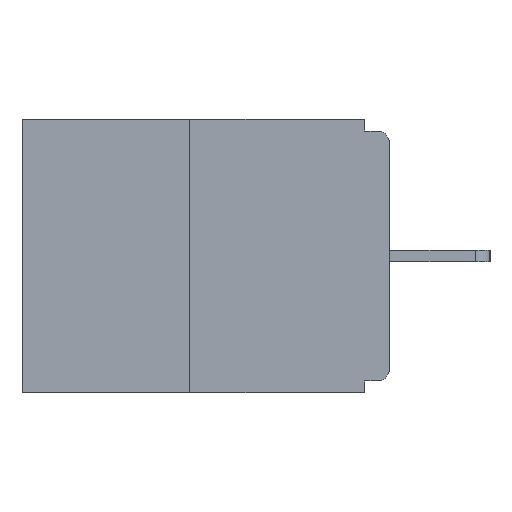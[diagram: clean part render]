
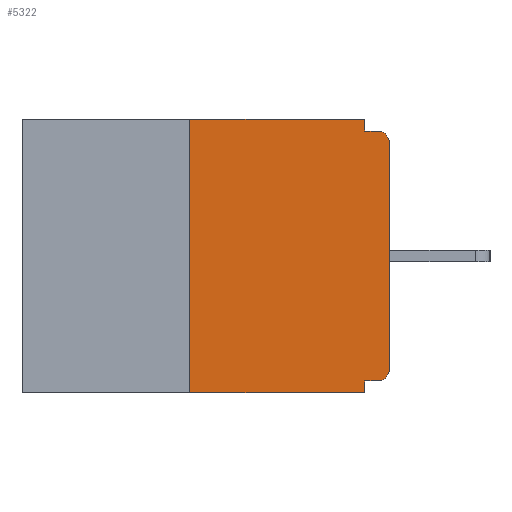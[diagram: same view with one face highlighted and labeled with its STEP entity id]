
A CAD part, left-side view. The second image highlights one B-rep face of the part: STEP entity #5322.
In plain terms, the highlighted planar face has unit normal (-1, 0, 0).
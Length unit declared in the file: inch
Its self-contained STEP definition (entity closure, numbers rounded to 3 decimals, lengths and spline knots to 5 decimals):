
#946 = ORIENTED_EDGE ( 'NONE', *, *, #2236, .F. ) ;
#1265 = CARTESIAN_POINT ( 'NONE',  ( 0., 0.46, 0. ) ) ;
#1408 = LINE ( 'NONE', #3053, #6652 ) ;
#1463 = DIRECTION ( 'NONE',  ( 0., 0., 1. ) ) ;
#1972 = EDGE_CURVE ( 'NONE', #5993, #9005, #5410, .T. ) ;
#2151 = DIRECTION ( 'NONE',  ( 0., -1., 0. ) ) ;
#2236 = EDGE_CURVE ( 'NONE', #11232, #6673, #1408, .T. ) ;
#2295 = CARTESIAN_POINT ( 'NONE',  ( 0., 0.015, -0.03 ) ) ;
#2318 = EDGE_CURVE ( 'NONE', #5993, #11232, #6804, .T. ) ;
#2478 = ORIENTED_EDGE ( 'NONE', *, *, #10260, .F. ) ;
#3053 = CARTESIAN_POINT ( 'NONE',  ( 0., 0.46, 0. ) ) ;
#3063 = EDGE_CURVE ( 'NONE', #16476, #9643, #3218, .T. ) ;
#3094 = CARTESIAN_POINT ( 'NONE',  ( 0., 0.031, -0.343 ) ) ;
#3218 = LINE ( 'NONE', #9120, #13230 ) ;
#3253 = EDGE_CURVE ( 'NONE', #18438, #9005, #6007, .T. ) ;
#3499 = ORIENTED_EDGE ( 'NONE', *, *, #1972, .T. ) ;
#3757 = AXIS2_PLACEMENT_3D ( 'NONE', #1265, #8915, #9019 ) ;
#3936 = DIRECTION ( 'NONE',  ( 0., 1., 0. ) ) ;
#4158 = EDGE_CURVE ( 'NONE', #9643, #14361, #6137, .T. ) ;
#5322 = ADVANCED_FACE ( 'NONE', ( #14964 ), #19705, .F. ) ;
#5410 = LINE ( 'NONE', #14597, #5956 ) ;
#5672 = CARTESIAN_POINT ( 'NONE',  ( 0., 0.25, 0. ) ) ;
#5891 = DIRECTION ( 'NONE',  ( 0., 0., -1. ) ) ;
#5905 = EDGE_CURVE ( 'NONE', #6673, #17529, #19989, .T. ) ;
#5956 = VECTOR ( 'NONE', #11450, 39.37008 ) ;
#5993 = VERTEX_POINT ( 'NONE', #13817 ) ;
#6007 = LINE ( 'NONE', #7640, #15175 ) ;
#6094 = DIRECTION ( 'NONE',  ( -1., 0., 0. ) ) ;
#6137 = CIRCLE ( 'NONE', #13275, 0.015 ) ;
#6310 = DIRECTION ( 'NONE',  ( 0., -1., 0. ) ) ;
#6607 = CARTESIAN_POINT ( 'NONE',  ( 0., 0.031, -0.015 ) ) ;
#6652 = VECTOR ( 'NONE', #6310, 39.37008 ) ;
#6673 = VERTEX_POINT ( 'NONE', #14785 ) ;
#6804 = LINE ( 'NONE', #14770, #10901 ) ;
#7176 = LINE ( 'NONE', #17956, #15007 ) ;
#7640 = CARTESIAN_POINT ( 'NONE',  ( 0., 0.031, -0.343 ) ) ;
#7729 = CARTESIAN_POINT ( 'NONE',  ( 0., 0.015, -0.313 ) ) ;
#8274 = ORIENTED_EDGE ( 'NONE', *, *, #4158, .T. ) ;
#8915 = DIRECTION ( 'NONE',  ( 1., 0., 0. ) ) ;
#9005 = VERTEX_POINT ( 'NONE', #3094 ) ;
#9019 = DIRECTION ( 'NONE',  ( 0., 0., -1. ) ) ;
#9120 = CARTESIAN_POINT ( 'NONE',  ( 0., 0., 0. ) ) ;
#9408 = VECTOR ( 'NONE', #2151, 39.37008 ) ;
#9628 = VERTEX_POINT ( 'NONE', #17994 ) ;
#9643 = VERTEX_POINT ( 'NONE', #19423 ) ;
#9787 = EDGE_CURVE ( 'NONE', #9628, #16476, #15399, .T. ) ;
#10260 = EDGE_CURVE ( 'NONE', #17529, #14361, #12190, .T. ) ;
#10830 = AXIS2_PLACEMENT_3D ( 'NONE', #7729, #6094, #5891 ) ;
#10844 = DIRECTION ( 'NONE',  ( 0., 0., -1. ) ) ;
#10901 = VECTOR ( 'NONE', #17667, 39.37008 ) ;
#11232 = VERTEX_POINT ( 'NONE', #5672 ) ;
#11450 = DIRECTION ( 'NONE',  ( 0., -1., 0. ) ) ;
#11486 = ORIENTED_EDGE ( 'NONE', *, *, #19213, .F. ) ;
#11955 = CARTESIAN_POINT ( 'NONE',  ( 0., 0.031, -0.328 ) ) ;
#12190 = LINE ( 'NONE', #18441, #9408 ) ;
#12256 = DIRECTION ( 'NONE',  ( 0., 0., -1. ) ) ;
#12392 = ORIENTED_EDGE ( 'NONE', *, *, #3253, .F. ) ;
#12699 = ORIENTED_EDGE ( 'NONE', *, *, #5905, .F. ) ;
#13208 = EDGE_LOOP ( 'NONE', ( #946, #16142, #3499, #12392, #11486, #18056, #15781, #8274, #2478, #12699 ) ) ;
#13230 = VECTOR ( 'NONE', #1463, 39.37008 ) ;
#13275 = AXIS2_PLACEMENT_3D ( 'NONE', #2295, #16008, #19504 ) ;
#13817 = CARTESIAN_POINT ( 'NONE',  ( 0., 0.25, -0.343 ) ) ;
#14361 = VERTEX_POINT ( 'NONE', #19850 ) ;
#14597 = CARTESIAN_POINT ( 'NONE',  ( 0., 0.46, -0.343 ) ) ;
#14770 = CARTESIAN_POINT ( 'NONE',  ( 0., 0.25, 0. ) ) ;
#14785 = CARTESIAN_POINT ( 'NONE',  ( 0., 0.031, 0. ) ) ;
#14964 = FACE_OUTER_BOUND ( 'NONE', #13208, .T. ) ;
#15007 = VECTOR ( 'NONE', #3936, 39.37008 ) ;
#15175 = VECTOR ( 'NONE', #12256, 39.37008 ) ;
#15399 = CIRCLE ( 'NONE', #10830, 0.015 ) ;
#15781 = ORIENTED_EDGE ( 'NONE', *, *, #3063, .T. ) ;
#16008 = DIRECTION ( 'NONE',  ( -1., 0., 0. ) ) ;
#16142 = ORIENTED_EDGE ( 'NONE', *, *, #2318, .F. ) ;
#16476 = VERTEX_POINT ( 'NONE', #19094 ) ;
#17529 = VERTEX_POINT ( 'NONE', #6607 ) ;
#17571 = VECTOR ( 'NONE', #10844, 39.37008 ) ;
#17667 = DIRECTION ( 'NONE',  ( 0., 0., 1. ) ) ;
#17956 = CARTESIAN_POINT ( 'NONE',  ( 0., 0., -0.328 ) ) ;
#17994 = CARTESIAN_POINT ( 'NONE',  ( 0., 0.015, -0.328 ) ) ;
#18056 = ORIENTED_EDGE ( 'NONE', *, *, #9787, .T. ) ;
#18438 = VERTEX_POINT ( 'NONE', #11955 ) ;
#18441 = CARTESIAN_POINT ( 'NONE',  ( 0., 0., -0.015 ) ) ;
#19094 = CARTESIAN_POINT ( 'NONE',  ( 0., 0., -0.313 ) ) ;
#19213 = EDGE_CURVE ( 'NONE', #9628, #18438, #7176, .T. ) ;
#19423 = CARTESIAN_POINT ( 'NONE',  ( 0., 0., -0.03 ) ) ;
#19504 = DIRECTION ( 'NONE',  ( 0., 0., -1. ) ) ;
#19705 = PLANE ( 'NONE',  #3757 ) ;
#19850 = CARTESIAN_POINT ( 'NONE',  ( 0., 0.015, -0.015 ) ) ;
#19989 = LINE ( 'NONE', #20080, #17571 ) ;
#20080 = CARTESIAN_POINT ( 'NONE',  ( 0., 0.031, 0. ) ) ;
